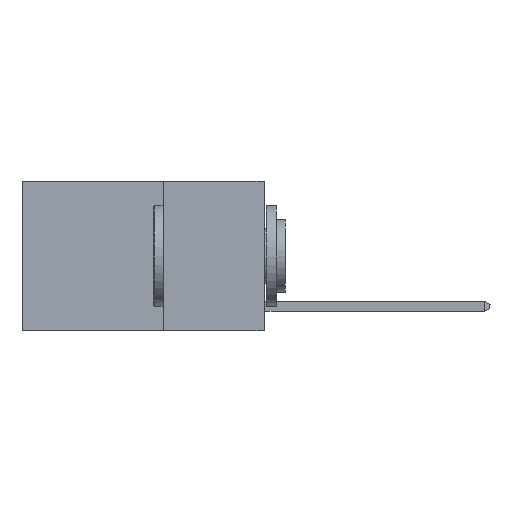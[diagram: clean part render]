
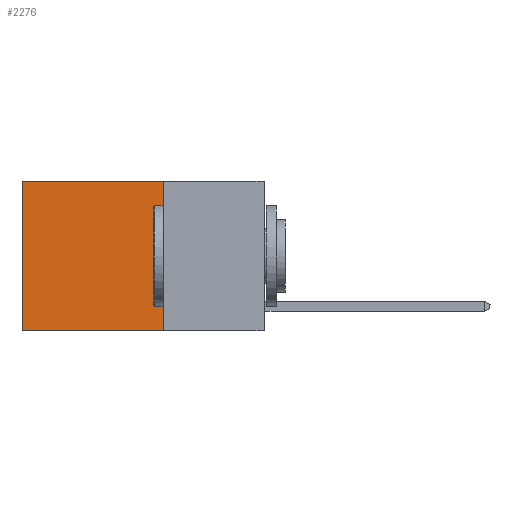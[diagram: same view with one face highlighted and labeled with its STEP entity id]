
A CAD part, left-side view. The second image highlights one B-rep face of the part: STEP entity #2276.
In plain terms, the highlighted planar face has unit normal (-1, 0, 0).
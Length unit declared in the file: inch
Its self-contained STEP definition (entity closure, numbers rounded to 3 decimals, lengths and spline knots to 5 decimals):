
#362 = ORIENTED_EDGE ( 'NONE', *, *, #18223, .F. ) ;
#665 = VERTEX_POINT ( 'NONE', #19562 ) ;
#1178 = VECTOR ( 'NONE', #24770, 39.37008 ) ;
#2276 = ADVANCED_FACE ( 'NONE', ( #18092 ), #13518, .F. ) ;
#3181 = AXIS2_PLACEMENT_3D ( 'NONE', #24070, #11482, #26165 ) ;
#3774 = CARTESIAN_POINT ( 'NONE',  ( 0.2625, 0.6, 0. ) ) ;
#6120 = LINE ( 'NONE', #3774, #1178 ) ;
#7333 = VECTOR ( 'NONE', #16522, 39.37008 ) ;
#8568 = EDGE_LOOP ( 'NONE', ( #17001, #362, #10508, #13056 ) ) ;
#8904 = VECTOR ( 'NONE', #26356, 39.37008 ) ;
#9563 = CARTESIAN_POINT ( 'NONE',  ( 0.2625, 0.25, 0. ) ) ;
#9597 = EDGE_CURVE ( 'NONE', #665, #23460, #15817, .T. ) ;
#10103 = LINE ( 'NONE', #22726, #19997 ) ;
#10508 = ORIENTED_EDGE ( 'NONE', *, *, #9597, .F. ) ;
#11482 = DIRECTION ( 'NONE',  ( 1., 0., 0. ) ) ;
#12248 = DIRECTION ( 'NONE',  ( 0., 1., 0. ) ) ;
#13056 = ORIENTED_EDGE ( 'NONE', *, *, #15751, .T. ) ;
#13116 = VERTEX_POINT ( 'NONE', #20189 ) ;
#13518 = PLANE ( 'NONE',  #3181 ) ;
#14418 = CARTESIAN_POINT ( 'NONE',  ( 0.2625, 0.25, -0.37 ) ) ;
#15751 = EDGE_CURVE ( 'NONE', #665, #26105, #10103, .T. ) ;
#15817 = LINE ( 'NONE', #9563, #8904 ) ;
#16302 = EDGE_CURVE ( 'NONE', #26105, #13116, #6120, .T. ) ;
#16522 = DIRECTION ( 'NONE',  ( 0., 1., 0. ) ) ;
#17001 = ORIENTED_EDGE ( 'NONE', *, *, #16302, .T. ) ;
#17877 = LINE ( 'NONE', #14418, #7333 ) ;
#18092 = FACE_OUTER_BOUND ( 'NONE', #8568, .T. ) ;
#18223 = EDGE_CURVE ( 'NONE', #23460, #13116, #17877, .T. ) ;
#19562 = CARTESIAN_POINT ( 'NONE',  ( 0.2625, 0.25, 0. ) ) ;
#19997 = VECTOR ( 'NONE', #12248, 39.37008 ) ;
#20189 = CARTESIAN_POINT ( 'NONE',  ( 0.2625, 0.6, -0.37 ) ) ;
#22726 = CARTESIAN_POINT ( 'NONE',  ( 0.2625, 0.25, 0. ) ) ;
#23100 = CARTESIAN_POINT ( 'NONE',  ( 0.2625, 0.25, -0.37 ) ) ;
#23460 = VERTEX_POINT ( 'NONE', #23100 ) ;
#24070 = CARTESIAN_POINT ( 'NONE',  ( 0.2625, 0.25, 0. ) ) ;
#24770 = DIRECTION ( 'NONE',  ( 0., 0., -1. ) ) ;
#26105 = VERTEX_POINT ( 'NONE', #26123 ) ;
#26123 = CARTESIAN_POINT ( 'NONE',  ( 0.2625, 0.6, 0. ) ) ;
#26165 = DIRECTION ( 'NONE',  ( 0., 0., -1. ) ) ;
#26356 = DIRECTION ( 'NONE',  ( 0., 0., -1. ) ) ;
